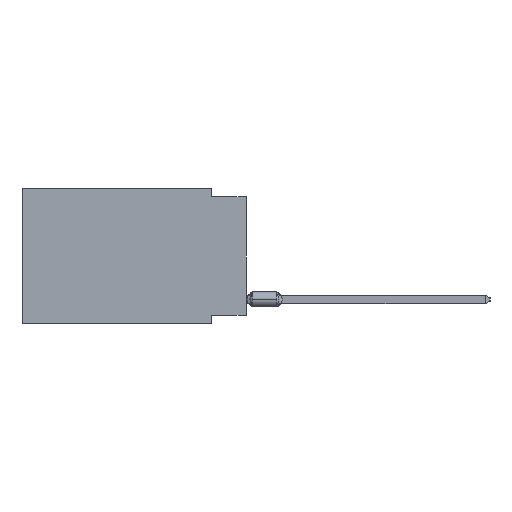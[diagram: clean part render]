
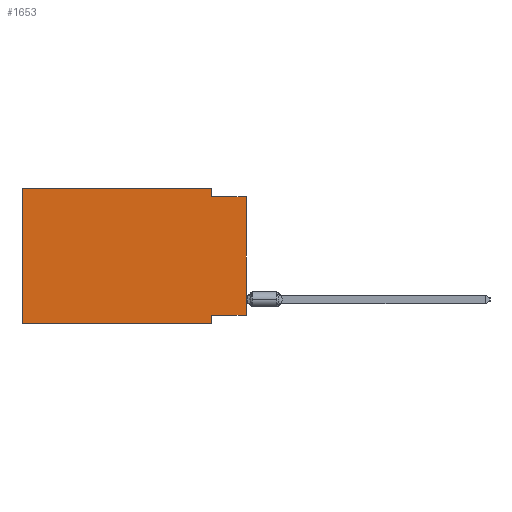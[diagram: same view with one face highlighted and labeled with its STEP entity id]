
A CAD part, left-side view. The second image highlights one B-rep face of the part: STEP entity #1653.
In plain terms, the highlighted planar face has unit normal (-1, 0, 0).
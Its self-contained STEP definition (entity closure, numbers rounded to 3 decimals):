
#943 = DIRECTION ( 'NONE',  ( 0., -1., 0. ) ) ;
#1653 = ADVANCED_FACE ( 'NONE', ( #37634 ), #57242, .F. ) ;
#3347 = DIRECTION ( 'NONE',  ( 0., 0., -1. ) ) ;
#3352 = CARTESIAN_POINT ( 'NONE',  ( 0., 16.383, 0. ) ) ;
#5212 = ORIENTED_EDGE ( 'NONE', *, *, #64913, .F. ) ;
#8964 = LINE ( 'NONE', #68649, #12343 ) ;
#9359 = ORIENTED_EDGE ( 'NONE', *, *, #19177, .T. ) ;
#12343 = VECTOR ( 'NONE', #943, 1000. ) ;
#12446 = DIRECTION ( 'NONE',  ( 0., -1., 0. ) ) ;
#13023 = CARTESIAN_POINT ( 'NONE',  ( 0., 2.54, 0. ) ) ;
#13649 = VERTEX_POINT ( 'NONE', #36871 ) ;
#15119 = EDGE_CURVE ( 'NONE', #78560, #41244, #61018, .T. ) ;
#15492 = EDGE_CURVE ( 'NONE', #41244, #52813, #33319, .T. ) ;
#16047 = VECTOR ( 'NONE', #71692, 1000. ) ;
#16387 = CARTESIAN_POINT ( 'NONE',  ( 0., 0., 0. ) ) ;
#18096 = EDGE_CURVE ( 'NONE', #13649, #23055, #77840, .T. ) ;
#19177 = EDGE_CURVE ( 'NONE', #32709, #23055, #8964, .T. ) ;
#19343 = ORIENTED_EDGE ( 'NONE', *, *, #18096, .F. ) ;
#21749 = DIRECTION ( 'NONE',  ( 0., 0., 1. ) ) ;
#23055 = VERTEX_POINT ( 'NONE', #77010 ) ;
#24818 = DIRECTION ( 'NONE',  ( 0., 0., -1. ) ) ;
#27166 = DIRECTION ( 'NONE',  ( 0., 0., -1. ) ) ;
#28549 = VECTOR ( 'NONE', #12446, 1000. ) ;
#30334 = LINE ( 'NONE', #85154, #60758 ) ;
#30965 = AXIS2_PLACEMENT_3D ( 'NONE', #77314, #38066, #3347 ) ;
#32709 = VERTEX_POINT ( 'NONE', #80206 ) ;
#33319 = LINE ( 'NONE', #60486, #61872 ) ;
#33669 = ORIENTED_EDGE ( 'NONE', *, *, #45307, .F. ) ;
#36871 = CARTESIAN_POINT ( 'NONE',  ( 0., 2.54, -9.271 ) ) ;
#37634 = FACE_OUTER_BOUND ( 'NONE', #53522, .T. ) ;
#38066 = DIRECTION ( 'NONE',  ( 1., 0., 0. ) ) ;
#38235 = VERTEX_POINT ( 'NONE', #81865 ) ;
#38348 = VECTOR ( 'NONE', #21749, 1000. ) ;
#41244 = VERTEX_POINT ( 'NONE', #85193 ) ;
#41959 = VECTOR ( 'NONE', #27166, 1000. ) ;
#43967 = CARTESIAN_POINT ( 'NONE',  ( 0., 2.54, -9.906 ) ) ;
#44060 = CARTESIAN_POINT ( 'NONE',  ( 0., 16.383, 0. ) ) ;
#45307 = EDGE_CURVE ( 'NONE', #32709, #59879, #50740, .T. ) ;
#46715 = LINE ( 'NONE', #54293, #28549 ) ;
#50740 = LINE ( 'NONE', #44060, #16047 ) ;
#52813 = VERTEX_POINT ( 'NONE', #60175 ) ;
#53522 = EDGE_LOOP ( 'NONE', ( #57969, #64855, #71070, #69133, #33669, #9359, #19343, #5212 ) ) ;
#54293 = CARTESIAN_POINT ( 'NONE',  ( 0., 16.383, 0. ) ) ;
#57242 = PLANE ( 'NONE',  #30965 ) ;
#57969 = ORIENTED_EDGE ( 'NONE', *, *, #59395, .T. ) ;
#59395 = EDGE_CURVE ( 'NONE', #38235, #52813, #77415, .T. ) ;
#59879 = VERTEX_POINT ( 'NONE', #3352 ) ;
#60175 = CARTESIAN_POINT ( 'NONE',  ( 0., 0., -0.635 ) ) ;
#60486 = CARTESIAN_POINT ( 'NONE',  ( 0., 0., -0.635 ) ) ;
#60523 = VECTOR ( 'NONE', #24818, 1000. ) ;
#60758 = VECTOR ( 'NONE', #70883, 1000. ) ;
#61018 = LINE ( 'NONE', #79772, #41959 ) ;
#61872 = VECTOR ( 'NONE', #87696, 1000. ) ;
#64855 = ORIENTED_EDGE ( 'NONE', *, *, #15492, .F. ) ;
#64913 = EDGE_CURVE ( 'NONE', #38235, #13649, #30334, .T. ) ;
#68649 = CARTESIAN_POINT ( 'NONE',  ( 0., 16.383, -9.906 ) ) ;
#69133 = ORIENTED_EDGE ( 'NONE', *, *, #79215, .F. ) ;
#70883 = DIRECTION ( 'NONE',  ( 0., 1., 0. ) ) ;
#71070 = ORIENTED_EDGE ( 'NONE', *, *, #15119, .F. ) ;
#71692 = DIRECTION ( 'NONE',  ( 0., 0., 1. ) ) ;
#77010 = CARTESIAN_POINT ( 'NONE',  ( 0., 2.54, -9.906 ) ) ;
#77314 = CARTESIAN_POINT ( 'NONE',  ( 0., 16.383, 0. ) ) ;
#77415 = LINE ( 'NONE', #16387, #38348 ) ;
#77840 = LINE ( 'NONE', #43967, #60523 ) ;
#78560 = VERTEX_POINT ( 'NONE', #13023 ) ;
#79215 = EDGE_CURVE ( 'NONE', #59879, #78560, #46715, .T. ) ;
#79772 = CARTESIAN_POINT ( 'NONE',  ( 0., 2.54, 0. ) ) ;
#80206 = CARTESIAN_POINT ( 'NONE',  ( 0., 16.383, -9.906 ) ) ;
#81865 = CARTESIAN_POINT ( 'NONE',  ( 0., 0., -9.271 ) ) ;
#85154 = CARTESIAN_POINT ( 'NONE',  ( 0., 0., -9.271 ) ) ;
#85193 = CARTESIAN_POINT ( 'NONE',  ( 0., 2.54, -0.635 ) ) ;
#87696 = DIRECTION ( 'NONE',  ( 0., -1., 0. ) ) ;
